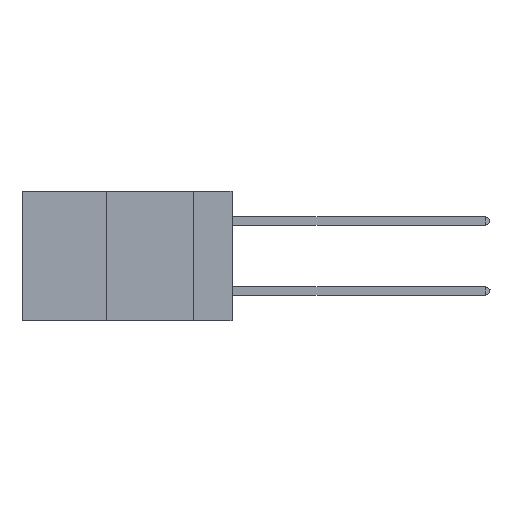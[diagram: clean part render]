
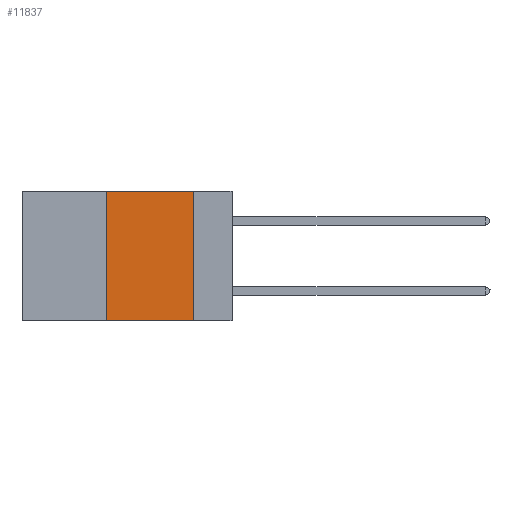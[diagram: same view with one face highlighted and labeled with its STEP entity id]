
A CAD part, left-side view. The second image highlights one B-rep face of the part: STEP entity #11837.
In plain terms, the highlighted planar face has unit normal (-1, 0, 0).
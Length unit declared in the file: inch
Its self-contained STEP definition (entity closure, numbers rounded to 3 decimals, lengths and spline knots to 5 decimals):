
#79 = ORIENTED_EDGE ( 'NONE', *, *, #8767, .F. ) ;
#198 = DIRECTION ( 'NONE',  ( 0., 0., -1. ) ) ;
#885 = VERTEX_POINT ( 'NONE', #21520 ) ;
#2379 = VECTOR ( 'NONE', #7642, 39.37008 ) ;
#3973 = CARTESIAN_POINT ( 'NONE',  ( 0., 0.36, 0. ) ) ;
#5364 = VERTEX_POINT ( 'NONE', #28028 ) ;
#5479 = ORIENTED_EDGE ( 'NONE', *, *, #10139, .F. ) ;
#7146 = CARTESIAN_POINT ( 'NONE',  ( 0., 0.36, 0. ) ) ;
#7642 = DIRECTION ( 'NONE',  ( 0., -1., 0. ) ) ;
#8597 = VERTEX_POINT ( 'NONE', #7146 ) ;
#8767 = EDGE_CURVE ( 'NONE', #8597, #5364, #19058, .T. ) ;
#10139 = EDGE_CURVE ( 'NONE', #885, #8597, #26327, .T. ) ;
#11423 = EDGE_CURVE ( 'NONE', #5364, #32985, #22975, .T. ) ;
#11837 = ADVANCED_FACE ( 'NONE', ( #21744 ), #33602, .F. ) ;
#12361 = VECTOR ( 'NONE', #198, 39.37008 ) ;
#12888 = VECTOR ( 'NONE', #22642, 39.37008 ) ;
#13134 = EDGE_CURVE ( 'NONE', #885, #32985, #16140, .T. ) ;
#14501 = EDGE_LOOP ( 'NONE', ( #24832, #79, #5479, #31668 ) ) ;
#16140 = LINE ( 'NONE', #20007, #12888 ) ;
#16534 = VECTOR ( 'NONE', #30501, 39.37008 ) ;
#17939 = AXIS2_PLACEMENT_3D ( 'NONE', #31088, #26046, #18399 ) ;
#18399 = DIRECTION ( 'NONE',  ( 0., 0., -1. ) ) ;
#18662 = CARTESIAN_POINT ( 'NONE',  ( 0., 0.11, 0. ) ) ;
#19058 = LINE ( 'NONE', #28390, #2379 ) ;
#20007 = CARTESIAN_POINT ( 'NONE',  ( 0., 0.6, -0.37 ) ) ;
#21520 = CARTESIAN_POINT ( 'NONE',  ( 0., 0.36, -0.37 ) ) ;
#21744 = FACE_OUTER_BOUND ( 'NONE', #14501, .T. ) ;
#22642 = DIRECTION ( 'NONE',  ( 0., -1., 0. ) ) ;
#22975 = LINE ( 'NONE', #18662, #12361 ) ;
#24832 = ORIENTED_EDGE ( 'NONE', *, *, #11423, .F. ) ;
#25009 = CARTESIAN_POINT ( 'NONE',  ( 0., 0.11, -0.37 ) ) ;
#26046 = DIRECTION ( 'NONE',  ( 1., 0., 0. ) ) ;
#26327 = LINE ( 'NONE', #3973, #16534 ) ;
#28028 = CARTESIAN_POINT ( 'NONE',  ( 0., 0.11, 0. ) ) ;
#28390 = CARTESIAN_POINT ( 'NONE',  ( 0., 0.6, 0. ) ) ;
#30501 = DIRECTION ( 'NONE',  ( 0., 0., 1. ) ) ;
#31088 = CARTESIAN_POINT ( 'NONE',  ( 0., 0.6, 0. ) ) ;
#31668 = ORIENTED_EDGE ( 'NONE', *, *, #13134, .T. ) ;
#32985 = VERTEX_POINT ( 'NONE', #25009 ) ;
#33602 = PLANE ( 'NONE',  #17939 ) ;
